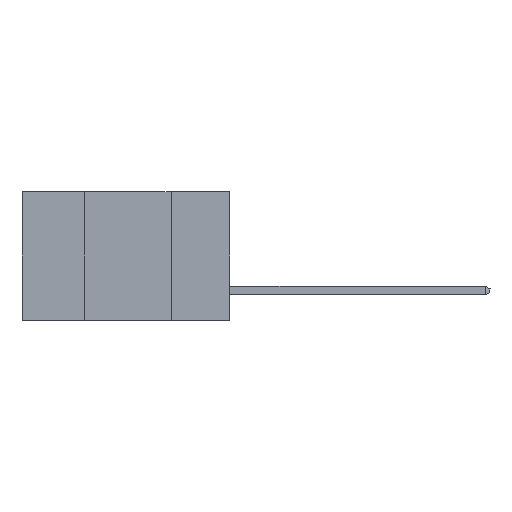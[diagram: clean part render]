
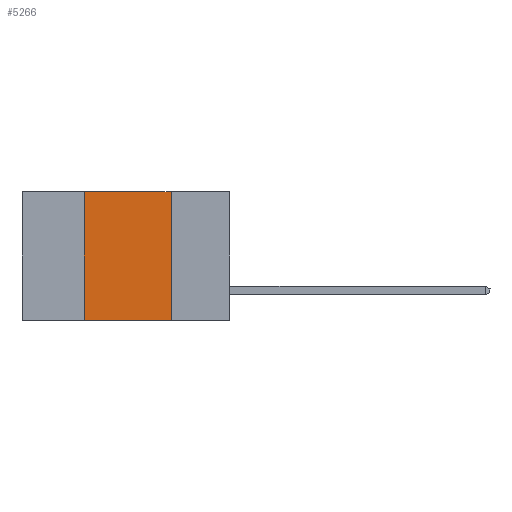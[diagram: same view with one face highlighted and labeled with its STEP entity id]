
A CAD part, left-side view. The second image highlights one B-rep face of the part: STEP entity #5266.
In plain terms, the highlighted planar face has unit normal (-1, 0, 0).
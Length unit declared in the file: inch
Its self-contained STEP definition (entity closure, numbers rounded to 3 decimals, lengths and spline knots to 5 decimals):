
#87 = CARTESIAN_POINT ( 'NONE',  ( 0., 0.17, -0.37 ) ) ;
#396 = VERTEX_POINT ( 'NONE', #9350 ) ;
#1663 = VERTEX_POINT ( 'NONE', #10307 ) ;
#1704 = DIRECTION ( 'NONE',  ( 0., -1., 0. ) ) ;
#1751 = ORIENTED_EDGE ( 'NONE', *, *, #6441, .F. ) ;
#1753 = LINE ( 'NONE', #9710, #7695 ) ;
#1880 = DIRECTION ( 'NONE',  ( 0., 0., 1. ) ) ;
#2003 = VECTOR ( 'NONE', #9128, 39.37008 ) ;
#2125 = DIRECTION ( 'NONE',  ( 1., 0., 0. ) ) ;
#2565 = EDGE_CURVE ( 'NONE', #3041, #1663, #2633, .T. ) ;
#2633 = LINE ( 'NONE', #10579, #11623 ) ;
#2972 = FACE_OUTER_BOUND ( 'NONE', #7330, .T. ) ;
#3041 = VERTEX_POINT ( 'NONE', #4774 ) ;
#3241 = DIRECTION ( 'NONE',  ( 0., 0., -1. ) ) ;
#4057 = LINE ( 'NONE', #87, #2003 ) ;
#4590 = ORIENTED_EDGE ( 'NONE', *, *, #12696, .F. ) ;
#4774 = CARTESIAN_POINT ( 'NONE',  ( 0., 0.42, -0.37 ) ) ;
#5005 = CARTESIAN_POINT ( 'NONE',  ( 0., 0.6, 0. ) ) ;
#5266 = ADVANCED_FACE ( 'NONE', ( #2972 ), #6957, .F. ) ;
#5408 = ORIENTED_EDGE ( 'NONE', *, *, #12413, .F. ) ;
#5782 = DIRECTION ( 'NONE',  ( 0., -1., 0. ) ) ;
#6441 = EDGE_CURVE ( 'NONE', #3041, #6763, #1753, .T. ) ;
#6763 = VERTEX_POINT ( 'NONE', #7295 ) ;
#6957 = PLANE ( 'NONE',  #9184 ) ;
#7295 = CARTESIAN_POINT ( 'NONE',  ( 0., 0.42, 0. ) ) ;
#7330 = EDGE_LOOP ( 'NONE', ( #4590, #5408, #1751, #10874 ) ) ;
#7583 = CARTESIAN_POINT ( 'NONE',  ( 0., 0.6, 0. ) ) ;
#7695 = VECTOR ( 'NONE', #1880, 39.37008 ) ;
#9128 = DIRECTION ( 'NONE',  ( 0., 0., -1. ) ) ;
#9184 = AXIS2_PLACEMENT_3D ( 'NONE', #5005, #2125, #3241 ) ;
#9350 = CARTESIAN_POINT ( 'NONE',  ( 0., 0.17, 0. ) ) ;
#9710 = CARTESIAN_POINT ( 'NONE',  ( 0., 0.42, -0.37 ) ) ;
#10307 = CARTESIAN_POINT ( 'NONE',  ( 0., 0.17, -0.37 ) ) ;
#10579 = CARTESIAN_POINT ( 'NONE',  ( 0., 0.6, -0.37 ) ) ;
#10630 = LINE ( 'NONE', #7583, #11354 ) ;
#10874 = ORIENTED_EDGE ( 'NONE', *, *, #2565, .T. ) ;
#11354 = VECTOR ( 'NONE', #1704, 39.37008 ) ;
#11623 = VECTOR ( 'NONE', #5782, 39.37008 ) ;
#12413 = EDGE_CURVE ( 'NONE', #6763, #396, #10630, .T. ) ;
#12696 = EDGE_CURVE ( 'NONE', #396, #1663, #4057, .T. ) ;
